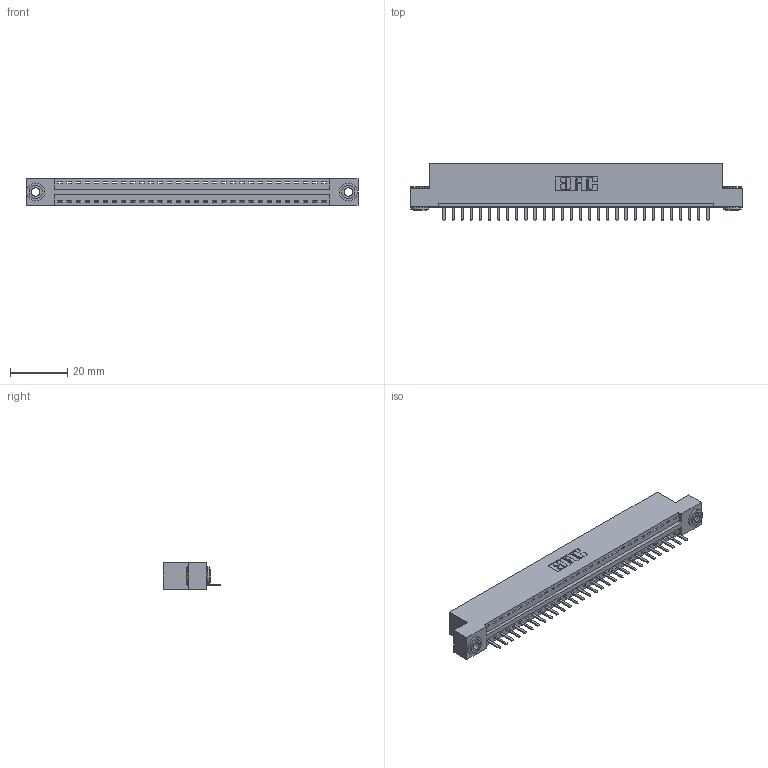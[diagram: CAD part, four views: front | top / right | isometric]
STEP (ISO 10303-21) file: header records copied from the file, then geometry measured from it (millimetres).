
FILE_DESCRIPTION (( 'STEP AP203' ), '1' );
FILE_NAME ('346-030-520-103.STEP', '2018-08-22T04:12:25', ( '' ), ( '' ), 'SwSTEP 2.0', 'SolidWorks 2016', '' );
FILE_SCHEMA (( 'CONFIG_CONTROL_DESIGN' ));
Length unit declared in the file: inch
Products named in the file (4): 346 Part_Flush Mounting Lugs - 0.156 Dia-TH; 345-292-001_345-293-120; 345-250-002_345-250-002-102; 346-030-520-103
Assembly tree (33 placements, depth 2):
  346-030-520-103
    346 Part_Flush Mounting Lugs - 0.156 Dia-TH
    345-292-001_345-293-120  x30
    345-250-002_345-250-002-102  x2
Bounding box: 115.82 x 20.02 x 9.4 mm (x, y, z)
Volume: 10937.3 mm3; surface area: 13471.9 mm2
Topology: 33 solids, 33 shells, 2020 faces, 5925 edges, 3866 vertices
Faces by surface type: plane 1346, cylinder 666, cone 8
Entity records: 20998 total; most frequent: CARTESIAN_POINT 3593, ORIENTED_EDGE 3538, DIRECTION 3203, EDGE_CURVE 1769, VECTOR 1489, LINE 1489, VERTEX_POINT 1174, AXIS2_PLACEMENT_3D 857
